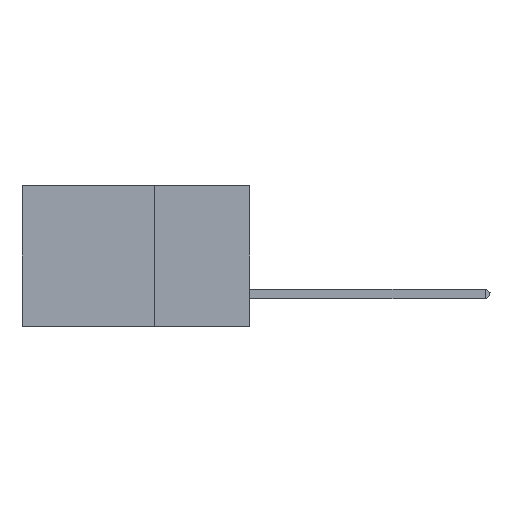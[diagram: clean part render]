
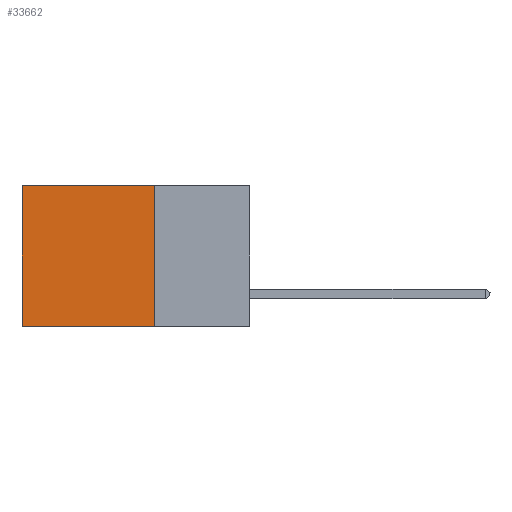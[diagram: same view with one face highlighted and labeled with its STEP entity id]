
A CAD part, left-side view. The second image highlights one B-rep face of the part: STEP entity #33662.
In plain terms, the highlighted planar face has unit normal (-1, 0, 0).
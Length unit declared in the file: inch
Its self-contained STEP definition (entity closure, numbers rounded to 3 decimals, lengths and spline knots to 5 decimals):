
#1648 = ORIENTED_EDGE ( 'NONE', *, *, #45328, .F. ) ;
#2591 = DIRECTION ( 'NONE',  ( 0., 1., 0. ) ) ;
#3122 = EDGE_CURVE ( 'NONE', #21945, #33179, #44985, .T. ) ;
#3628 = CARTESIAN_POINT ( 'NONE',  ( 0.2875, 0.25, -0.37 ) ) ;
#4899 = PLANE ( 'NONE',  #44873 ) ;
#5093 = VECTOR ( 'NONE', #32896, 39.37008 ) ;
#6153 = CARTESIAN_POINT ( 'NONE',  ( 0.2875, 0.6, 0. ) ) ;
#9130 = ORIENTED_EDGE ( 'NONE', *, *, #33350, .T. ) ;
#11912 = LINE ( 'NONE', #25217, #15428 ) ;
#12022 = VERTEX_POINT ( 'NONE', #25810 ) ;
#15428 = VECTOR ( 'NONE', #2591, 39.37008 ) ;
#17957 = EDGE_CURVE ( 'NONE', #24070, #12022, #21070, .T. ) ;
#20809 = VECTOR ( 'NONE', #30173, 39.37008 ) ;
#21070 = LINE ( 'NONE', #39972, #5093 ) ;
#21510 = EDGE_LOOP ( 'NONE', ( #23458, #1648, #33275, #9130 ) ) ;
#21945 = VERTEX_POINT ( 'NONE', #6153 ) ;
#22578 = CARTESIAN_POINT ( 'NONE',  ( 0.2875, 0.6, 0. ) ) ;
#23458 = ORIENTED_EDGE ( 'NONE', *, *, #3122, .T. ) ;
#23871 = CARTESIAN_POINT ( 'NONE',  ( 0.2875, 0.25, 0. ) ) ;
#24070 = VERTEX_POINT ( 'NONE', #23871 ) ;
#24916 = VECTOR ( 'NONE', #30866, 39.37008 ) ;
#25217 = CARTESIAN_POINT ( 'NONE',  ( 0.2875, 0.25, 0. ) ) ;
#25450 = FACE_OUTER_BOUND ( 'NONE', #21510, .T. ) ;
#25810 = CARTESIAN_POINT ( 'NONE',  ( 0.2875, 0.25, -0.37 ) ) ;
#26674 = LINE ( 'NONE', #3628, #24916 ) ;
#30173 = DIRECTION ( 'NONE',  ( 0., 0., -1. ) ) ;
#30866 = DIRECTION ( 'NONE',  ( 0., 1., 0. ) ) ;
#31324 = DIRECTION ( 'NONE',  ( 1., 0., 0. ) ) ;
#32346 = CARTESIAN_POINT ( 'NONE',  ( 0.2875, 0.6, -0.37 ) ) ;
#32896 = DIRECTION ( 'NONE',  ( 0., 0., -1. ) ) ;
#33179 = VERTEX_POINT ( 'NONE', #32346 ) ;
#33275 = ORIENTED_EDGE ( 'NONE', *, *, #17957, .F. ) ;
#33350 = EDGE_CURVE ( 'NONE', #24070, #21945, #11912, .T. ) ;
#33662 = ADVANCED_FACE ( 'NONE', ( #25450 ), #4899, .F. ) ;
#39972 = CARTESIAN_POINT ( 'NONE',  ( 0.2875, 0.25, 0. ) ) ;
#42511 = CARTESIAN_POINT ( 'NONE',  ( 0.2875, 0.25, 0. ) ) ;
#42997 = DIRECTION ( 'NONE',  ( 0., 0., -1. ) ) ;
#44873 = AXIS2_PLACEMENT_3D ( 'NONE', #42511, #31324, #42997 ) ;
#44985 = LINE ( 'NONE', #22578, #20809 ) ;
#45328 = EDGE_CURVE ( 'NONE', #12022, #33179, #26674, .T. ) ;
